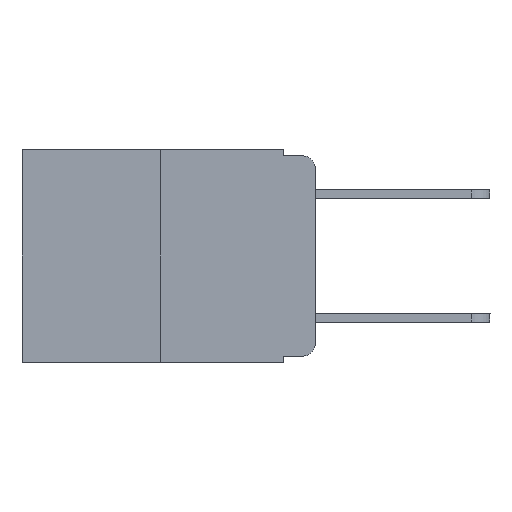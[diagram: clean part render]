
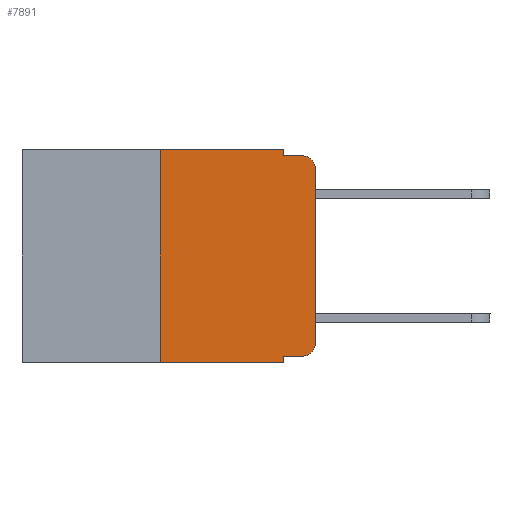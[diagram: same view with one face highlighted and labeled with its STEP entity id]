
A CAD part, left-side view. The second image highlights one B-rep face of the part: STEP entity #7891.
In plain terms, the highlighted planar face has unit normal (-1, 0, 0).
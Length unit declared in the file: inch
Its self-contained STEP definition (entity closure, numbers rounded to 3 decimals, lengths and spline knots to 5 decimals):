
#159 = DIRECTION ( 'NONE',  ( 1., 0., 0. ) ) ;
#209 = CARTESIAN_POINT ( 'NONE',  ( 0., 0.051, 0. ) ) ;
#217 = CARTESIAN_POINT ( 'NONE',  ( 0., 0.473, 0. ) ) ;
#309 = DIRECTION ( 'NONE',  ( 0., 0., -1. ) ) ;
#500 = VERTEX_POINT ( 'NONE', #11636 ) ;
#727 = EDGE_CURVE ( 'NONE', #5502, #1969, #5684, .T. ) ;
#948 = CARTESIAN_POINT ( 'NONE',  ( 0., 0.473, 0. ) ) ;
#1001 = DIRECTION ( 'NONE',  ( 0., -1., 0. ) ) ;
#1224 = VECTOR ( 'NONE', #14080, 39.37008 ) ;
#1250 = DIRECTION ( 'NONE',  ( 0., -1., 0. ) ) ;
#1318 = ORIENTED_EDGE ( 'NONE', *, *, #6522, .T. ) ;
#1373 = ORIENTED_EDGE ( 'NONE', *, *, #12037, .F. ) ;
#1969 = VERTEX_POINT ( 'NONE', #12586 ) ;
#1987 = LINE ( 'NONE', #7944, #15781 ) ;
#2271 = VERTEX_POINT ( 'NONE', #13453 ) ;
#2328 = VECTOR ( 'NONE', #4988, 39.37008 ) ;
#2395 = EDGE_CURVE ( 'NONE', #16080, #9145, #4416, .T. ) ;
#2409 = CIRCLE ( 'NONE', #6013, 0.02 ) ;
#2526 = ORIENTED_EDGE ( 'NONE', *, *, #10713, .T. ) ;
#3100 = AXIS2_PLACEMENT_3D ( 'NONE', #10161, #9149, #309 ) ;
#3190 = LINE ( 'NONE', #209, #1224 ) ;
#3266 = CARTESIAN_POINT ( 'NONE',  ( 0., 0., -0.03 ) ) ;
#3493 = ORIENTED_EDGE ( 'NONE', *, *, #15678, .T. ) ;
#3705 = CARTESIAN_POINT ( 'NONE',  ( 0., 0.051, 0. ) ) ;
#3711 = LINE ( 'NONE', #948, #7843 ) ;
#3782 = ORIENTED_EDGE ( 'NONE', *, *, #8403, .T. ) ;
#4226 = DIRECTION ( 'NONE',  ( 0., 0., 1. ) ) ;
#4416 = LINE ( 'NONE', #5965, #11738 ) ;
#4765 = VECTOR ( 'NONE', #8365, 39.37008 ) ;
#4988 = DIRECTION ( 'NONE',  ( 0., 0., -1. ) ) ;
#5174 = DIRECTION ( 'NONE',  ( 0., 0., -1. ) ) ;
#5225 = ORIENTED_EDGE ( 'NONE', *, *, #2395, .F. ) ;
#5323 = DIRECTION ( 'NONE',  ( 0., 0., -1. ) ) ;
#5502 = VERTEX_POINT ( 'NONE', #16184 ) ;
#5684 = LINE ( 'NONE', #3705, #2328 ) ;
#5965 = CARTESIAN_POINT ( 'NONE',  ( 0., 0.051, -0.01 ) ) ;
#6013 = AXIS2_PLACEMENT_3D ( 'NONE', #15270, #7728, #5323 ) ;
#6116 = ORIENTED_EDGE ( 'NONE', *, *, #10756, .F. ) ;
#6522 = EDGE_CURVE ( 'NONE', #2271, #7783, #12524, .T. ) ;
#7728 = DIRECTION ( 'NONE',  ( -1., 0., 0. ) ) ;
#7783 = VERTEX_POINT ( 'NONE', #12508 ) ;
#7843 = VECTOR ( 'NONE', #14911, 39.37008 ) ;
#7891 = ADVANCED_FACE ( 'NONE', ( #15010 ), #12731, .F. ) ;
#7944 = CARTESIAN_POINT ( 'NONE',  ( 0., 0.473, -0.343 ) ) ;
#8352 = ORIENTED_EDGE ( 'NONE', *, *, #727, .F. ) ;
#8365 = DIRECTION ( 'NONE',  ( 0., 0., 1. ) ) ;
#8403 = EDGE_CURVE ( 'NONE', #12771, #1969, #1987, .T. ) ;
#8671 = DIRECTION ( 'NONE',  ( 0., -1., 0. ) ) ;
#8837 = CARTESIAN_POINT ( 'NONE',  ( 0., 0.051, -0.01 ) ) ;
#9145 = VERTEX_POINT ( 'NONE', #12056 ) ;
#9149 = DIRECTION ( 'NONE',  ( -1., 0., 0. ) ) ;
#9529 = VECTOR ( 'NONE', #4226, 39.37008 ) ;
#9822 = EDGE_CURVE ( 'NONE', #12771, #500, #11338, .T. ) ;
#9905 = ORIENTED_EDGE ( 'NONE', *, *, #16016, .T. ) ;
#10161 = CARTESIAN_POINT ( 'NONE',  ( 0., 0.02, -0.313 ) ) ;
#10274 = CARTESIAN_POINT ( 'NONE',  ( 0., 0.25, -0.343 ) ) ;
#10713 = EDGE_CURVE ( 'NONE', #13160, #9145, #2409, .T. ) ;
#10756 = EDGE_CURVE ( 'NONE', #14155, #16080, #3190, .T. ) ;
#11303 = LINE ( 'NONE', #12455, #15033 ) ;
#11338 = LINE ( 'NONE', #13556, #4765 ) ;
#11636 = CARTESIAN_POINT ( 'NONE',  ( 0., 0.25, 0. ) ) ;
#11685 = AXIS2_PLACEMENT_3D ( 'NONE', #217, #159, #5174 ) ;
#11738 = VECTOR ( 'NONE', #1001, 39.37008 ) ;
#12037 = EDGE_CURVE ( 'NONE', #500, #14155, #3711, .T. ) ;
#12056 = CARTESIAN_POINT ( 'NONE',  ( 0., 0.02, -0.01 ) ) ;
#12455 = CARTESIAN_POINT ( 'NONE',  ( 0., 0.051, -0.333 ) ) ;
#12508 = CARTESIAN_POINT ( 'NONE',  ( 0., 0., -0.313 ) ) ;
#12524 = CIRCLE ( 'NONE', #3100, 0.02 ) ;
#12586 = CARTESIAN_POINT ( 'NONE',  ( 0., 0.051, -0.343 ) ) ;
#12731 = PLANE ( 'NONE',  #11685 ) ;
#12771 = VERTEX_POINT ( 'NONE', #10274 ) ;
#12899 = CARTESIAN_POINT ( 'NONE',  ( 0., 0., 0. ) ) ;
#12973 = EDGE_LOOP ( 'NONE', ( #3493, #2526, #5225, #6116, #1373, #14755, #3782, #8352, #9905, #1318 ) ) ;
#13099 = LINE ( 'NONE', #12899, #9529 ) ;
#13160 = VERTEX_POINT ( 'NONE', #3266 ) ;
#13453 = CARTESIAN_POINT ( 'NONE',  ( 0., 0.02, -0.333 ) ) ;
#13556 = CARTESIAN_POINT ( 'NONE',  ( 0., 0.25, 0. ) ) ;
#14080 = DIRECTION ( 'NONE',  ( 0., 0., -1. ) ) ;
#14155 = VERTEX_POINT ( 'NONE', #14266 ) ;
#14266 = CARTESIAN_POINT ( 'NONE',  ( 0., 0.051, 0. ) ) ;
#14755 = ORIENTED_EDGE ( 'NONE', *, *, #9822, .F. ) ;
#14911 = DIRECTION ( 'NONE',  ( 0., -1., 0. ) ) ;
#15010 = FACE_OUTER_BOUND ( 'NONE', #12973, .T. ) ;
#15033 = VECTOR ( 'NONE', #8671, 39.37008 ) ;
#15270 = CARTESIAN_POINT ( 'NONE',  ( 0., 0.02, -0.03 ) ) ;
#15678 = EDGE_CURVE ( 'NONE', #7783, #13160, #13099, .T. ) ;
#15781 = VECTOR ( 'NONE', #1250, 39.37008 ) ;
#16016 = EDGE_CURVE ( 'NONE', #5502, #2271, #11303, .T. ) ;
#16080 = VERTEX_POINT ( 'NONE', #8837 ) ;
#16184 = CARTESIAN_POINT ( 'NONE',  ( 0., 0.051, -0.333 ) ) ;
